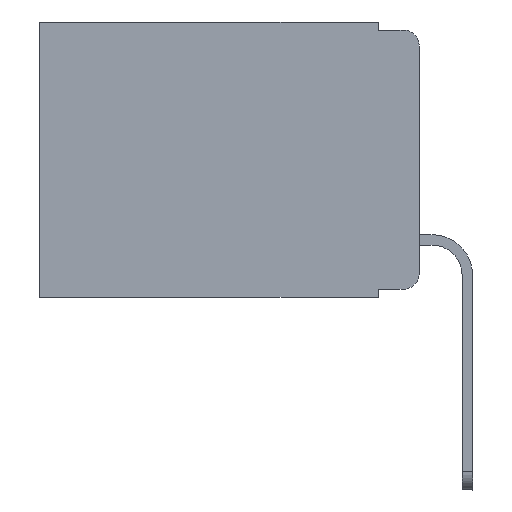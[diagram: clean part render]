
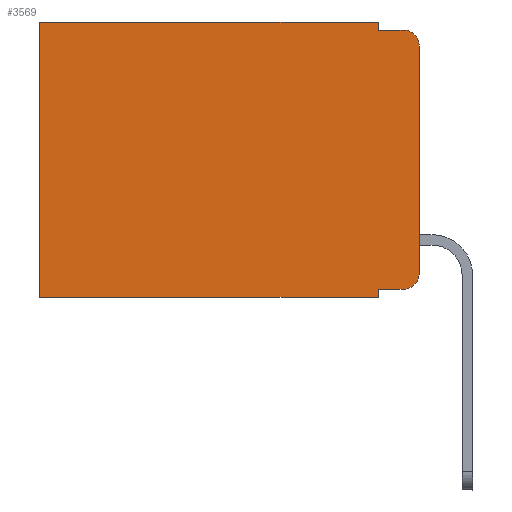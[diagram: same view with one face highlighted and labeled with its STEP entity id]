
A CAD part, left-side view. The second image highlights one B-rep face of the part: STEP entity #3569.
In plain terms, the highlighted planar face has unit normal (-1, 0, 0).
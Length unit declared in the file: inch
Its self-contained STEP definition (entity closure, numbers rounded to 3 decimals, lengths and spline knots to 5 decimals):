
#97 = CARTESIAN_POINT ( 'NONE',  ( 0.298, 0.051, -0.01 ) ) ;
#109 = CARTESIAN_POINT ( 'NONE',  ( 0.298, 0., 0. ) ) ;
#481 = VECTOR ( 'NONE', #3087, 39.37008 ) ;
#1804 = ORIENTED_EDGE ( 'NONE', *, *, #12708, .T. ) ;
#1872 = CIRCLE ( 'NONE', #11327, 0.02 ) ;
#1967 = DIRECTION ( 'NONE',  ( -1., 0., 0. ) ) ;
#2176 = EDGE_CURVE ( 'NONE', #12214, #2619, #12620, .T. ) ;
#2282 = LINE ( 'NONE', #8531, #11862 ) ;
#2409 = ORIENTED_EDGE ( 'NONE', *, *, #7599, .F. ) ;
#2494 = DIRECTION ( 'NONE',  ( 1., 0., 0. ) ) ;
#2619 = VERTEX_POINT ( 'NONE', #3392 ) ;
#2691 = EDGE_CURVE ( 'NONE', #9374, #9372, #16104, .T. ) ;
#2756 = CARTESIAN_POINT ( 'NONE',  ( 0.298, 0.051, 0. ) ) ;
#3087 = DIRECTION ( 'NONE',  ( 0., 0., -1. ) ) ;
#3164 = VECTOR ( 'NONE', #11399, 39.37008 ) ;
#3392 = CARTESIAN_POINT ( 'NONE',  ( 0.298, 0.02, -0.01 ) ) ;
#3569 = ADVANCED_FACE ( 'NONE', ( #13042 ), #11518, .F. ) ;
#4445 = DIRECTION ( 'NONE',  ( -1., 0., 0. ) ) ;
#4494 = CARTESIAN_POINT ( 'NONE',  ( 0.298, 0.02, -0.03 ) ) ;
#4709 = VERTEX_POINT ( 'NONE', #9362 ) ;
#4800 = LINE ( 'NONE', #12659, #3164 ) ;
#4872 = ORIENTED_EDGE ( 'NONE', *, *, #13144, .F. ) ;
#4926 = ORIENTED_EDGE ( 'NONE', *, *, #11570, .F. ) ;
#4967 = CARTESIAN_POINT ( 'NONE',  ( 0.298, 0.051, -0.333 ) ) ;
#5101 = ORIENTED_EDGE ( 'NONE', *, *, #9018, .T. ) ;
#5390 = DIRECTION ( 'NONE',  ( 0., -1., 0. ) ) ;
#5796 = VECTOR ( 'NONE', #8641, 39.37008 ) ;
#5831 = CARTESIAN_POINT ( 'NONE',  ( 0.298, 0.051, 0. ) ) ;
#5979 = CARTESIAN_POINT ( 'NONE',  ( 0.298, 0., -0.03 ) ) ;
#6107 = DIRECTION ( 'NONE',  ( 0., -1., 0. ) ) ;
#6372 = VERTEX_POINT ( 'NONE', #7169 ) ;
#6490 = CARTESIAN_POINT ( 'NONE',  ( 0.298, 0.051, -0.333 ) ) ;
#6806 = LINE ( 'NONE', #10780, #481 ) ;
#7075 = EDGE_CURVE ( 'NONE', #9398, #2619, #1872, .T. ) ;
#7169 = CARTESIAN_POINT ( 'NONE',  ( 0.298, 0.473, 0. ) ) ;
#7223 = CARTESIAN_POINT ( 'NONE',  ( 0.298, 0.02, -0.313 ) ) ;
#7599 = EDGE_CURVE ( 'NONE', #9372, #14708, #2282, .T. ) ;
#7751 = VECTOR ( 'NONE', #5390, 39.37008 ) ;
#8324 = VECTOR ( 'NONE', #11105, 39.37008 ) ;
#8366 = VERTEX_POINT ( 'NONE', #8807 ) ;
#8531 = CARTESIAN_POINT ( 'NONE',  ( 0.298, 0., -0.343 ) ) ;
#8582 = DIRECTION ( 'NONE',  ( 0., 0., -1. ) ) ;
#8641 = DIRECTION ( 'NONE',  ( 0., 0., -1. ) ) ;
#8778 = ORIENTED_EDGE ( 'NONE', *, *, #2691, .F. ) ;
#8807 = CARTESIAN_POINT ( 'NONE',  ( 0.298, 0., -0.313 ) ) ;
#9018 = EDGE_CURVE ( 'NONE', #9374, #4709, #10632, .T. ) ;
#9170 = ORIENTED_EDGE ( 'NONE', *, *, #7075, .T. ) ;
#9362 = CARTESIAN_POINT ( 'NONE',  ( 0.298, 0.02, -0.333 ) ) ;
#9372 = VERTEX_POINT ( 'NONE', #12655 ) ;
#9374 = VERTEX_POINT ( 'NONE', #4967 ) ;
#9398 = VERTEX_POINT ( 'NONE', #5979 ) ;
#9413 = LINE ( 'NONE', #13639, #8324 ) ;
#9420 = ORIENTED_EDGE ( 'NONE', *, *, #2176, .F. ) ;
#9615 = EDGE_CURVE ( 'NONE', #6372, #14708, #6806, .T. ) ;
#10071 = ORIENTED_EDGE ( 'NONE', *, *, #9615, .T. ) ;
#10129 = DIRECTION ( 'NONE',  ( 0., 1., 0. ) ) ;
#10201 = AXIS2_PLACEMENT_3D ( 'NONE', #7223, #4445, #12052 ) ;
#10632 = LINE ( 'NONE', #6490, #7751 ) ;
#10780 = CARTESIAN_POINT ( 'NONE',  ( 0.298, 0.473, 0. ) ) ;
#11105 = DIRECTION ( 'NONE',  ( 0., 0., -1. ) ) ;
#11327 = AXIS2_PLACEMENT_3D ( 'NONE', #4494, #1967, #15936 ) ;
#11363 = CARTESIAN_POINT ( 'NONE',  ( 0.298, 0.051, -0.01 ) ) ;
#11399 = DIRECTION ( 'NONE',  ( 0., 1., 0. ) ) ;
#11453 = LINE ( 'NONE', #16651, #12954 ) ;
#11518 = PLANE ( 'NONE',  #13526 ) ;
#11570 = EDGE_CURVE ( 'NONE', #9398, #8366, #11453, .T. ) ;
#11862 = VECTOR ( 'NONE', #10129, 39.37008 ) ;
#12052 = DIRECTION ( 'NONE',  ( 0., 0., -1. ) ) ;
#12086 = CIRCLE ( 'NONE', #10201, 0.02 ) ;
#12214 = VERTEX_POINT ( 'NONE', #97 ) ;
#12348 = EDGE_LOOP ( 'NONE', ( #4926, #9170, #9420, #4872, #12795, #10071, #2409, #8778, #5101, #1804 ) ) ;
#12354 = EDGE_CURVE ( 'NONE', #12560, #6372, #4800, .T. ) ;
#12560 = VERTEX_POINT ( 'NONE', #2756 ) ;
#12620 = LINE ( 'NONE', #11363, #12641 ) ;
#12641 = VECTOR ( 'NONE', #6107, 39.37008 ) ;
#12655 = CARTESIAN_POINT ( 'NONE',  ( 0.298, 0.051, -0.343 ) ) ;
#12659 = CARTESIAN_POINT ( 'NONE',  ( 0.298, 0., 0. ) ) ;
#12708 = EDGE_CURVE ( 'NONE', #4709, #8366, #12086, .T. ) ;
#12795 = ORIENTED_EDGE ( 'NONE', *, *, #12354, .T. ) ;
#12796 = DIRECTION ( 'NONE',  ( 0., 0., -1. ) ) ;
#12954 = VECTOR ( 'NONE', #8582, 39.37008 ) ;
#13042 = FACE_OUTER_BOUND ( 'NONE', #12348, .T. ) ;
#13144 = EDGE_CURVE ( 'NONE', #12560, #12214, #9413, .T. ) ;
#13526 = AXIS2_PLACEMENT_3D ( 'NONE', #109, #2494, #12796 ) ;
#13639 = CARTESIAN_POINT ( 'NONE',  ( 0.298, 0.051, 0. ) ) ;
#14090 = CARTESIAN_POINT ( 'NONE',  ( 0.298, 0.473, -0.343 ) ) ;
#14708 = VERTEX_POINT ( 'NONE', #14090 ) ;
#15936 = DIRECTION ( 'NONE',  ( 0., 0., -1. ) ) ;
#16104 = LINE ( 'NONE', #5831, #5796 ) ;
#16651 = CARTESIAN_POINT ( 'NONE',  ( 0.298, 0., 0. ) ) ;
